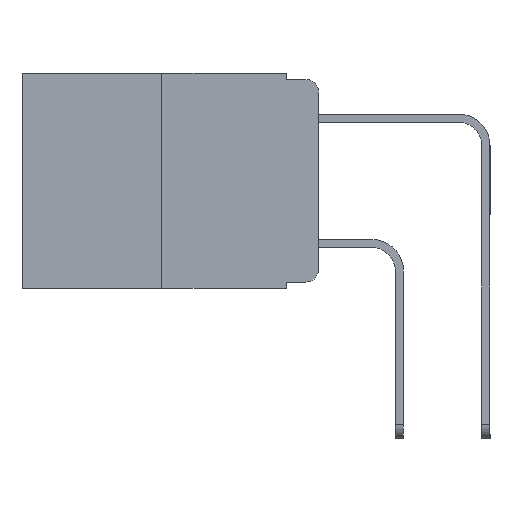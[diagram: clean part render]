
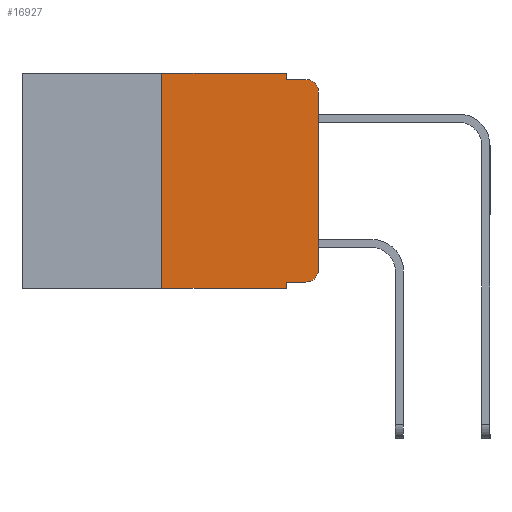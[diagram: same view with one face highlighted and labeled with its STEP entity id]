
A CAD part, left-side view. The second image highlights one B-rep face of the part: STEP entity #16927.
In plain terms, the highlighted planar face has unit normal (-1, 0, 0).
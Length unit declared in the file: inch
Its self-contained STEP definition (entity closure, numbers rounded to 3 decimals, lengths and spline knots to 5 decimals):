
#139 = FACE_OUTER_BOUND ( 'NONE', #8880, .T. ) ;
#174 = VECTOR ( 'NONE', #19112, 39.37008 ) ;
#204 = ORIENTED_EDGE ( 'NONE', *, *, #19058, .F. ) ;
#322 = CARTESIAN_POINT ( 'NONE',  ( 0., 0.473, 0. ) ) ;
#754 = LINE ( 'NONE', #322, #174 ) ;
#772 = VERTEX_POINT ( 'NONE', #21878 ) ;
#943 = VERTEX_POINT ( 'NONE', #3786 ) ;
#1039 = ORIENTED_EDGE ( 'NONE', *, *, #17553, .T. ) ;
#1255 = DIRECTION ( 'NONE',  ( 0., 0., 1. ) ) ;
#1362 = DIRECTION ( 'NONE',  ( 1., 0., 0. ) ) ;
#2350 = CARTESIAN_POINT ( 'NONE',  ( 0., 0.051, -0.343 ) ) ;
#2439 = VECTOR ( 'NONE', #2474, 39.37008 ) ;
#2474 = DIRECTION ( 'NONE',  ( 0., 0., -1. ) ) ;
#2536 = VERTEX_POINT ( 'NONE', #23014 ) ;
#2972 = EDGE_CURVE ( 'NONE', #21290, #772, #23339, .T. ) ;
#3203 = DIRECTION ( 'NONE',  ( -1., 0., 0. ) ) ;
#3323 = AXIS2_PLACEMENT_3D ( 'NONE', #12687, #1362, #14537 ) ;
#3703 = VERTEX_POINT ( 'NONE', #2350 ) ;
#3786 = CARTESIAN_POINT ( 'NONE',  ( 0., 0.02, -0.01 ) ) ;
#4062 = ORIENTED_EDGE ( 'NONE', *, *, #12523, .T. ) ;
#5200 = ORIENTED_EDGE ( 'NONE', *, *, #13204, .T. ) ;
#5260 = DIRECTION ( 'NONE',  ( 0., 0., -1. ) ) ;
#5541 = DIRECTION ( 'NONE',  ( 0., -1., 0. ) ) ;
#5678 = VERTEX_POINT ( 'NONE', #15824 ) ;
#6092 = ORIENTED_EDGE ( 'NONE', *, *, #2972, .F. ) ;
#6192 = VECTOR ( 'NONE', #5541, 39.37008 ) ;
#6223 = CARTESIAN_POINT ( 'NONE',  ( 0., 0.051, 0. ) ) ;
#6565 = AXIS2_PLACEMENT_3D ( 'NONE', #14493, #3203, #16380 ) ;
#6756 = VECTOR ( 'NONE', #14375, 39.37008 ) ;
#7409 = LINE ( 'NONE', #14903, #6192 ) ;
#7493 = CIRCLE ( 'NONE', #15299, 0.02 ) ;
#7597 = ORIENTED_EDGE ( 'NONE', *, *, #10583, .F. ) ;
#7945 = DIRECTION ( 'NONE',  ( -1., 0., 0. ) ) ;
#8236 = ORIENTED_EDGE ( 'NONE', *, *, #16597, .T. ) ;
#8259 = VERTEX_POINT ( 'NONE', #14466 ) ;
#8405 = VECTOR ( 'NONE', #5260, 39.37008 ) ;
#8761 = CARTESIAN_POINT ( 'NONE',  ( 0., 0.473, -0.343 ) ) ;
#8880 = EDGE_LOOP ( 'NONE', ( #1039, #22782, #204, #7597, #18707, #6092, #5200, #14334, #4062, #8236 ) ) ;
#10373 = DIRECTION ( 'NONE',  ( 0., -1., 0. ) ) ;
#10583 = EDGE_CURVE ( 'NONE', #8259, #14808, #22419, .T. ) ;
#10681 = CARTESIAN_POINT ( 'NONE',  ( 0., 0.25, -0.343 ) ) ;
#10848 = EDGE_CURVE ( 'NONE', #15499, #943, #16573, .T. ) ;
#11798 = LINE ( 'NONE', #8761, #6756 ) ;
#12523 = EDGE_CURVE ( 'NONE', #15232, #2536, #23189, .T. ) ;
#12687 = CARTESIAN_POINT ( 'NONE',  ( 0., 0.473, 0. ) ) ;
#13204 = EDGE_CURVE ( 'NONE', #21290, #3703, #11798, .T. ) ;
#13212 = DIRECTION ( 'NONE',  ( 0., 0., 1. ) ) ;
#13421 = VECTOR ( 'NONE', #13212, 39.37008 ) ;
#14334 = ORIENTED_EDGE ( 'NONE', *, *, #21382, .F. ) ;
#14375 = DIRECTION ( 'NONE',  ( 0., -1., 0. ) ) ;
#14466 = CARTESIAN_POINT ( 'NONE',  ( 0., 0.051, 0. ) ) ;
#14493 = CARTESIAN_POINT ( 'NONE',  ( 0., 0.02, -0.03 ) ) ;
#14537 = DIRECTION ( 'NONE',  ( 0., 0., -1. ) ) ;
#14783 = VECTOR ( 'NONE', #1255, 39.37008 ) ;
#14808 = VERTEX_POINT ( 'NONE', #21072 ) ;
#14903 = CARTESIAN_POINT ( 'NONE',  ( 0., 0.051, -0.01 ) ) ;
#15232 = VERTEX_POINT ( 'NONE', #16938 ) ;
#15299 = AXIS2_PLACEMENT_3D ( 'NONE', #19131, #7945, #20982 ) ;
#15343 = EDGE_CURVE ( 'NONE', #772, #8259, #754, .T. ) ;
#15499 = VERTEX_POINT ( 'NONE', #17643 ) ;
#15824 = CARTESIAN_POINT ( 'NONE',  ( 0., 0., -0.313 ) ) ;
#16227 = CARTESIAN_POINT ( 'NONE',  ( 0., 0., 0. ) ) ;
#16380 = DIRECTION ( 'NONE',  ( 0., 0., -1. ) ) ;
#16573 = CIRCLE ( 'NONE', #6565, 0.02 ) ;
#16597 = EDGE_CURVE ( 'NONE', #2536, #5678, #7493, .T. ) ;
#16927 = ADVANCED_FACE ( 'NONE', ( #139 ), #21876, .F. ) ;
#16938 = CARTESIAN_POINT ( 'NONE',  ( 0., 0.051, -0.333 ) ) ;
#17553 = EDGE_CURVE ( 'NONE', #5678, #15499, #19737, .T. ) ;
#17643 = CARTESIAN_POINT ( 'NONE',  ( 0., 0., -0.03 ) ) ;
#17772 = CARTESIAN_POINT ( 'NONE',  ( 0., 0.051, -0.333 ) ) ;
#18211 = VECTOR ( 'NONE', #10373, 39.37008 ) ;
#18399 = CARTESIAN_POINT ( 'NONE',  ( 0., 0.051, 0. ) ) ;
#18707 = ORIENTED_EDGE ( 'NONE', *, *, #15343, .F. ) ;
#18756 = CARTESIAN_POINT ( 'NONE',  ( 0., 0.25, 0. ) ) ;
#18912 = LINE ( 'NONE', #18399, #8405 ) ;
#19058 = EDGE_CURVE ( 'NONE', #14808, #943, #7409, .T. ) ;
#19112 = DIRECTION ( 'NONE',  ( 0., -1., 0. ) ) ;
#19131 = CARTESIAN_POINT ( 'NONE',  ( 0., 0.02, -0.313 ) ) ;
#19737 = LINE ( 'NONE', #16227, #14783 ) ;
#20982 = DIRECTION ( 'NONE',  ( 0., 0., -1. ) ) ;
#21072 = CARTESIAN_POINT ( 'NONE',  ( 0., 0.051, -0.01 ) ) ;
#21290 = VERTEX_POINT ( 'NONE', #10681 ) ;
#21382 = EDGE_CURVE ( 'NONE', #15232, #3703, #18912, .T. ) ;
#21876 = PLANE ( 'NONE',  #3323 ) ;
#21878 = CARTESIAN_POINT ( 'NONE',  ( 0., 0.25, 0. ) ) ;
#22419 = LINE ( 'NONE', #6223, #2439 ) ;
#22782 = ORIENTED_EDGE ( 'NONE', *, *, #10848, .T. ) ;
#23014 = CARTESIAN_POINT ( 'NONE',  ( 0., 0.02, -0.333 ) ) ;
#23189 = LINE ( 'NONE', #17772, #18211 ) ;
#23339 = LINE ( 'NONE', #18756, #13421 ) ;
